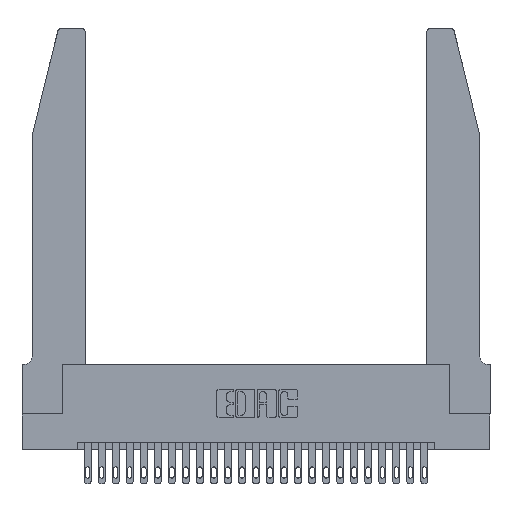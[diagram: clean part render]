
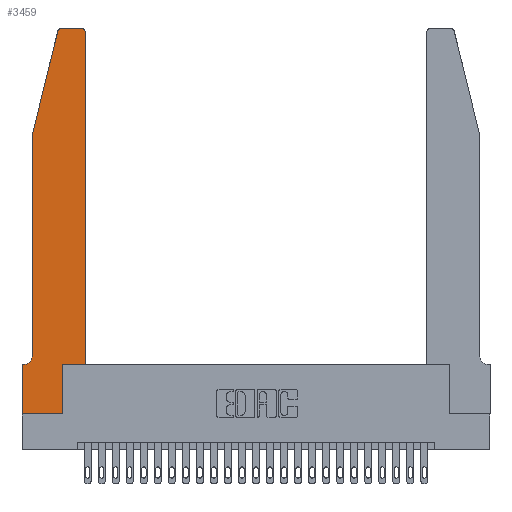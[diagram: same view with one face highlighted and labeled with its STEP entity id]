
A CAD part, top view. The second image highlights one B-rep face of the part: STEP entity #3459.
In plain terms, the highlighted planar face has unit normal (0, 0, 1).
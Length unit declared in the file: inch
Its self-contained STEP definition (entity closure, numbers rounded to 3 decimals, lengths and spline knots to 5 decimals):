
#176 = DIRECTION ( 'NONE',  ( -0.239, -0.971, 0. ) ) ;
#262 = DIRECTION ( 'NONE',  ( 0., -1., 0. ) ) ;
#425 = AXIS2_PLACEMENT_3D ( 'NONE', #23842, #11517, #5531 ) ;
#931 = CIRCLE ( 'NONE', #425, 0.03 ) ;
#1017 = VERTEX_POINT ( 'NONE', #2468 ) ;
#1300 = EDGE_CURVE ( 'NONE', #23478, #26349, #5518, .T. ) ;
#1737 = ORIENTED_EDGE ( 'NONE', *, *, #19405, .T. ) ;
#1910 = VECTOR ( 'NONE', #262, 39.37008 ) ;
#2130 = EDGE_CURVE ( 'NONE', #15190, #17146, #11224, .T. ) ;
#2158 = VECTOR ( 'NONE', #12531, 39.37008 ) ;
#2468 = CARTESIAN_POINT ( 'NONE',  ( 0.25487, 2.72718, 0.37 ) ) ;
#2927 = VERTEX_POINT ( 'NONE', #7938 ) ;
#2959 = CARTESIAN_POINT ( 'NONE',  ( 0.2865, 0.35, 0.37 ) ) ;
#3329 = CARTESIAN_POINT ( 'NONE',  ( 0., 0.35, 0.37 ) ) ;
#3459 = ADVANCED_FACE ( 'NONE', ( #16614 ), #5285, .T. ) ;
#3969 = CIRCLE ( 'NONE', #25676, 0.07 ) ;
#4046 = DIRECTION ( 'NONE',  ( 1., 0., 0. ) ) ;
#4082 = CARTESIAN_POINT ( 'NONE',  ( 0.4505, 0.35, 0.37 ) ) ;
#4116 = VECTOR ( 'NONE', #17025, 39.37008 ) ;
#4646 = CARTESIAN_POINT ( 'NONE',  ( 0.0055, 0.42, 0.37 ) ) ;
#4823 = CARTESIAN_POINT ( 'NONE',  ( 0.2605, 2.75, 0.37 ) ) ;
#5083 = DIRECTION ( 'NONE',  ( 0., -1., 0. ) ) ;
#5285 = PLANE ( 'NONE',  #24562 ) ;
#5518 = LINE ( 'NONE', #12268, #7108 ) ;
#5531 = DIRECTION ( 'NONE',  ( 1., 0., 0. ) ) ;
#5624 = ORIENTED_EDGE ( 'NONE', *, *, #20573, .T. ) ;
#6427 = ORIENTED_EDGE ( 'NONE', *, *, #19097, .T. ) ;
#6887 = EDGE_CURVE ( 'NONE', #18738, #1017, #931, .T. ) ;
#7108 = VECTOR ( 'NONE', #4046, 39.37008 ) ;
#7557 = VECTOR ( 'NONE', #26453, 39.37008 ) ;
#7923 = DIRECTION ( 'NONE',  ( 1., 0., 0. ) ) ;
#7938 = CARTESIAN_POINT ( 'NONE',  ( 0.4505, 2.72, 0.37 ) ) ;
#7962 = VECTOR ( 'NONE', #13055, 39.37008 ) ;
#8657 = CARTESIAN_POINT ( 'NONE',  ( 0., 0., 0.37 ) ) ;
#9268 = ORIENTED_EDGE ( 'NONE', *, *, #22453, .T. ) ;
#9361 = ORIENTED_EDGE ( 'NONE', *, *, #17389, .T. ) ;
#10807 = LINE ( 'NONE', #4082, #4116 ) ;
#10973 = DIRECTION ( 'NONE',  ( 0., 0., -1. ) ) ;
#11224 = LINE ( 'NONE', #17325, #23111 ) ;
#11379 = CARTESIAN_POINT ( 'NONE',  ( 0.2865, 0., 0.37 ) ) ;
#11424 = ORIENTED_EDGE ( 'NONE', *, *, #20346, .T. ) ;
#11517 = DIRECTION ( 'NONE',  ( 0., 0., 1. ) ) ;
#12104 = ORIENTED_EDGE ( 'NONE', *, *, #23397, .T. ) ;
#12242 = VERTEX_POINT ( 'NONE', #20172 ) ;
#12268 = CARTESIAN_POINT ( 'NONE',  ( 0.4505, 0.35, 0.37 ) ) ;
#12531 = DIRECTION ( 'NONE',  ( 1., 0., 0. ) ) ;
#12546 = VECTOR ( 'NONE', #176, 39.37008 ) ;
#12625 = CARTESIAN_POINT ( 'NONE',  ( 0.0755, 2., 0.37 ) ) ;
#12655 = CARTESIAN_POINT ( 'NONE',  ( 0.0755, 2., 0.37 ) ) ;
#12734 = CARTESIAN_POINT ( 'NONE',  ( 0.284, 2.75, 0.37 ) ) ;
#12793 = CIRCLE ( 'NONE', #13486, 0.03 ) ;
#12877 = CARTESIAN_POINT ( 'NONE',  ( 0., 0., 0.37 ) ) ;
#12989 = LINE ( 'NONE', #24364, #7557 ) ;
#13055 = DIRECTION ( 'NONE',  ( -1., 0., 0. ) ) ;
#13421 = DIRECTION ( 'NONE',  ( 1., 0., 0. ) ) ;
#13486 = AXIS2_PLACEMENT_3D ( 'NONE', #22374, #20228, #7923 ) ;
#14154 = VERTEX_POINT ( 'NONE', #12877 ) ;
#14187 = DIRECTION ( 'NONE',  ( -1., 0., 0. ) ) ;
#15190 = VERTEX_POINT ( 'NONE', #12655 ) ;
#16297 = CARTESIAN_POINT ( 'NONE',  ( 0.0755, 0.42, 0.37 ) ) ;
#16614 = FACE_OUTER_BOUND ( 'NONE', #23779, .T. ) ;
#17025 = DIRECTION ( 'NONE',  ( 0., 1., 0. ) ) ;
#17078 = DIRECTION ( 'NONE',  ( -1., 0., 0. ) ) ;
#17079 = ORIENTED_EDGE ( 'NONE', *, *, #18391, .T. ) ;
#17146 = VERTEX_POINT ( 'NONE', #16297 ) ;
#17325 = CARTESIAN_POINT ( 'NONE',  ( 0.0755, 2., 0.37 ) ) ;
#17389 = EDGE_CURVE ( 'NONE', #1017, #15190, #18010, .T. ) ;
#17392 = ORIENTED_EDGE ( 'NONE', *, *, #19364, .T. ) ;
#17501 = ORIENTED_EDGE ( 'NONE', *, *, #1300, .T. ) ;
#17555 = DIRECTION ( 'NONE',  ( 0., 0., 1. ) ) ;
#17724 = CARTESIAN_POINT ( 'NONE',  ( 0.4505, 0.35, 0.37 ) ) ;
#18010 = LINE ( 'NONE', #12625, #12546 ) ;
#18391 = EDGE_CURVE ( 'NONE', #12242, #26560, #24724, .T. ) ;
#18499 = LINE ( 'NONE', #8657, #2158 ) ;
#18738 = VERTEX_POINT ( 'NONE', #12734 ) ;
#19097 = EDGE_CURVE ( 'NONE', #20385, #18738, #24368, .T. ) ;
#19364 = EDGE_CURVE ( 'NONE', #14154, #25603, #18499, .T. ) ;
#19405 = EDGE_CURVE ( 'NONE', #26560, #14154, #23061, .T. ) ;
#20172 = CARTESIAN_POINT ( 'NONE',  ( 0.0055, 0.35, 0.37 ) ) ;
#20228 = DIRECTION ( 'NONE',  ( 0., 0., 1. ) ) ;
#20346 = EDGE_CURVE ( 'NONE', #2927, #20385, #12793, .T. ) ;
#20385 = VERTEX_POINT ( 'NONE', #26528 ) ;
#20516 = CARTESIAN_POINT ( 'NONE',  ( 0., 0.35, 0.37 ) ) ;
#20573 = EDGE_CURVE ( 'NONE', #26349, #2927, #10807, .T. ) ;
#22374 = CARTESIAN_POINT ( 'NONE',  ( 0.4205, 2.72, 0.37 ) ) ;
#22453 = EDGE_CURVE ( 'NONE', #25603, #23478, #12989, .T. ) ;
#22457 = ORIENTED_EDGE ( 'NONE', *, *, #2130, .T. ) ;
#22767 = CARTESIAN_POINT ( 'NONE',  ( 0., 0., 0.37 ) ) ;
#23061 = LINE ( 'NONE', #22767, #1910 ) ;
#23111 = VECTOR ( 'NONE', #5083, 39.37008 ) ;
#23246 = ORIENTED_EDGE ( 'NONE', *, *, #6887, .T. ) ;
#23397 = EDGE_CURVE ( 'NONE', #17146, #12242, #3969, .T. ) ;
#23478 = VERTEX_POINT ( 'NONE', #2959 ) ;
#23779 = EDGE_LOOP ( 'NONE', ( #6427, #23246, #9361, #22457, #12104, #17079, #1737, #17392, #9268, #17501, #5624, #11424 ) ) ;
#23842 = CARTESIAN_POINT ( 'NONE',  ( 0.284, 2.72, 0.37 ) ) ;
#24350 = CARTESIAN_POINT ( 'NONE',  ( 0.0755, 0.35, 0.37 ) ) ;
#24364 = CARTESIAN_POINT ( 'NONE',  ( 0.2865, 0.35, 0.37 ) ) ;
#24368 = LINE ( 'NONE', #4823, #7962 ) ;
#24562 = AXIS2_PLACEMENT_3D ( 'NONE', #3329, #17555, #13421 ) ;
#24724 = LINE ( 'NONE', #24350, #25694 ) ;
#25603 = VERTEX_POINT ( 'NONE', #11379 ) ;
#25676 = AXIS2_PLACEMENT_3D ( 'NONE', #4646, #10973, #17078 ) ;
#25694 = VECTOR ( 'NONE', #14187, 39.37008 ) ;
#26349 = VERTEX_POINT ( 'NONE', #17724 ) ;
#26453 = DIRECTION ( 'NONE',  ( 0., 1., 0. ) ) ;
#26528 = CARTESIAN_POINT ( 'NONE',  ( 0.4205, 2.75, 0.37 ) ) ;
#26560 = VERTEX_POINT ( 'NONE', #20516 ) ;
